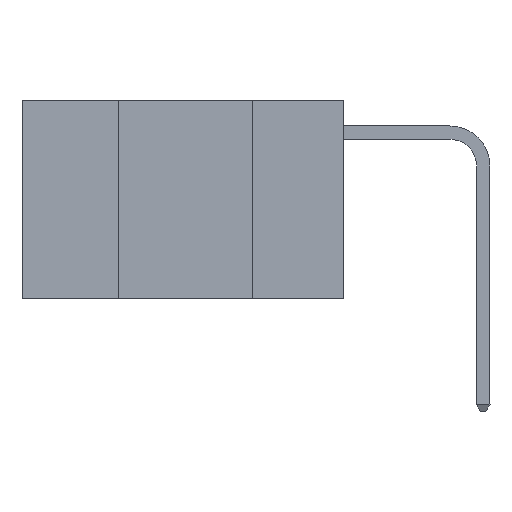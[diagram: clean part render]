
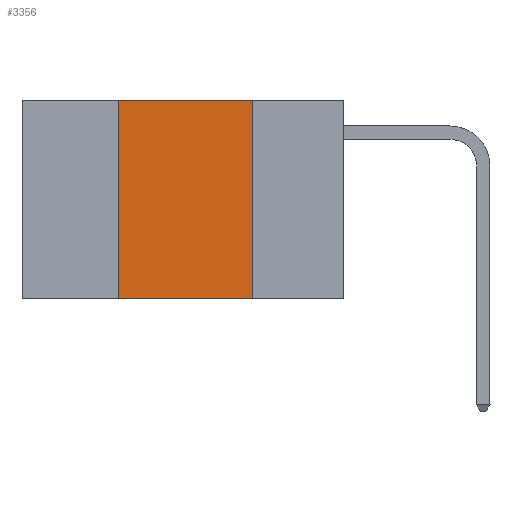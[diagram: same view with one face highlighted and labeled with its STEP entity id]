
A CAD part, left-side view. The second image highlights one B-rep face of the part: STEP entity #3356.
In plain terms, the highlighted planar face has unit normal (-1, 0, 0).
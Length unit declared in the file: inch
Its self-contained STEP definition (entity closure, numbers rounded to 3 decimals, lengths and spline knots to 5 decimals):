
#117 = CARTESIAN_POINT ( 'NONE',  ( 0., 0.42, 0. ) ) ;
#129 = CARTESIAN_POINT ( 'NONE',  ( 0., 0.42, -0.37 ) ) ;
#327 = CARTESIAN_POINT ( 'NONE',  ( 0., 0.42, 0. ) ) ;
#359 = CARTESIAN_POINT ( 'NONE',  ( 0., 0.6, 0. ) ) ;
#1071 = FACE_OUTER_BOUND ( 'NONE', #6526, .T. ) ;
#1314 = CARTESIAN_POINT ( 'NONE',  ( 0., 0.17, -0.37 ) ) ;
#1354 = AXIS2_PLACEMENT_3D ( 'NONE', #359, #8983, #2344 ) ;
#1477 = DIRECTION ( 'NONE',  ( 0., -1., 0. ) ) ;
#1841 = VERTEX_POINT ( 'NONE', #1314 ) ;
#1885 = CARTESIAN_POINT ( 'NONE',  ( 0., 0.6, 0. ) ) ;
#2344 = DIRECTION ( 'NONE',  ( 0., 0., -1. ) ) ;
#2558 = VECTOR ( 'NONE', #6173, 39.37008 ) ;
#2642 = DIRECTION ( 'NONE',  ( 0., -1., 0. ) ) ;
#3123 = LINE ( 'NONE', #6074, #2558 ) ;
#3356 = ADVANCED_FACE ( 'NONE', ( #1071 ), #6972, .F. ) ;
#4156 = LINE ( 'NONE', #327, #8657 ) ;
#4516 = EDGE_CURVE ( 'NONE', #4995, #1841, #6601, .T. ) ;
#4655 = EDGE_CURVE ( 'NONE', #4995, #7659, #4156, .T. ) ;
#4721 = VERTEX_POINT ( 'NONE', #8613 ) ;
#4898 = ORIENTED_EDGE ( 'NONE', *, *, #7515, .F. ) ;
#4995 = VERTEX_POINT ( 'NONE', #129 ) ;
#5035 = VECTOR ( 'NONE', #2642, 39.37008 ) ;
#5434 = ORIENTED_EDGE ( 'NONE', *, *, #4516, .T. ) ;
#5504 = ORIENTED_EDGE ( 'NONE', *, *, #8861, .F. ) ;
#5658 = ORIENTED_EDGE ( 'NONE', *, *, #4655, .F. ) ;
#5865 = CARTESIAN_POINT ( 'NONE',  ( 0., 0.6, -0.37 ) ) ;
#6074 = CARTESIAN_POINT ( 'NONE',  ( 0., 0.17, 0. ) ) ;
#6173 = DIRECTION ( 'NONE',  ( 0., 0., -1. ) ) ;
#6526 = EDGE_LOOP ( 'NONE', ( #5504, #4898, #5658, #5434 ) ) ;
#6601 = LINE ( 'NONE', #5865, #7432 ) ;
#6972 = PLANE ( 'NONE',  #1354 ) ;
#7024 = DIRECTION ( 'NONE',  ( 0., 0., 1. ) ) ;
#7432 = VECTOR ( 'NONE', #1477, 39.37008 ) ;
#7515 = EDGE_CURVE ( 'NONE', #7659, #4721, #9125, .T. ) ;
#7659 = VERTEX_POINT ( 'NONE', #117 ) ;
#8613 = CARTESIAN_POINT ( 'NONE',  ( 0., 0.17, 0. ) ) ;
#8657 = VECTOR ( 'NONE', #7024, 39.37008 ) ;
#8861 = EDGE_CURVE ( 'NONE', #4721, #1841, #3123, .T. ) ;
#8983 = DIRECTION ( 'NONE',  ( 1., 0., 0. ) ) ;
#9125 = LINE ( 'NONE', #1885, #5035 ) ;
